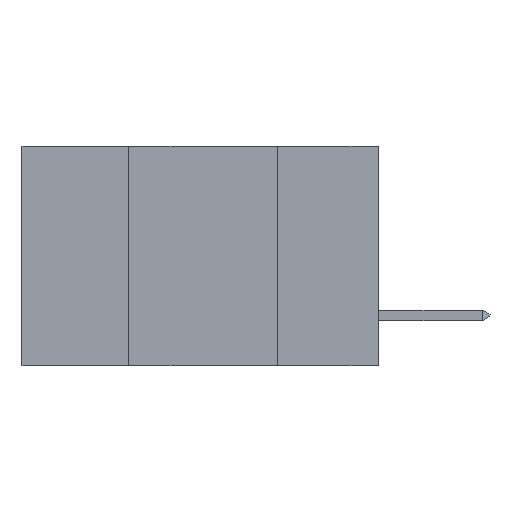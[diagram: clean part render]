
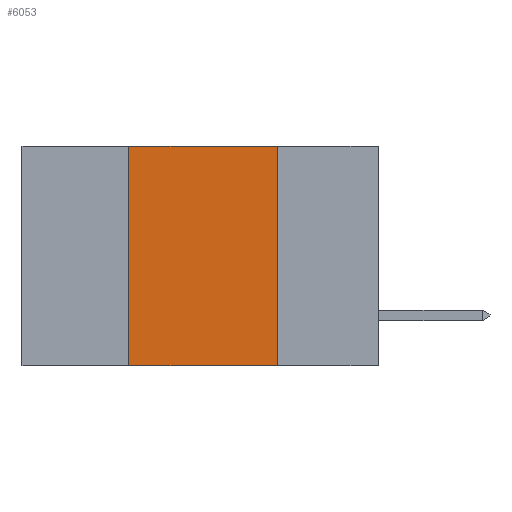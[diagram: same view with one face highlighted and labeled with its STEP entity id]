
A CAD part, left-side view. The second image highlights one B-rep face of the part: STEP entity #6053.
In plain terms, the highlighted planar face has unit normal (-1, 0, 0).
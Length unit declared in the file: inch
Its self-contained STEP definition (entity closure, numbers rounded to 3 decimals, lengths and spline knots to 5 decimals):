
#12 = PLANE ( 'NONE',  #1670 ) ;
#139 = DIRECTION ( 'NONE',  ( 0., 0., -1. ) ) ;
#550 = EDGE_LOOP ( 'NONE', ( #5480, #7150, #6984, #7961 ) ) ;
#715 = FACE_OUTER_BOUND ( 'NONE', #550, .T. ) ;
#751 = LINE ( 'NONE', #3348, #5535 ) ;
#835 = EDGE_CURVE ( 'NONE', #5811, #3957, #4386, .T. ) ;
#1568 = CARTESIAN_POINT ( 'NONE',  ( 0., 0.17, 0. ) ) ;
#1670 = AXIS2_PLACEMENT_3D ( 'NONE', #4110, #5445, #139 ) ;
#2428 = EDGE_CURVE ( 'NONE', #4372, #3389, #8267, .T. ) ;
#3314 = CARTESIAN_POINT ( 'NONE',  ( 0., 0.42, 0. ) ) ;
#3348 = CARTESIAN_POINT ( 'NONE',  ( 0., 0.6, 0. ) ) ;
#3389 = VERTEX_POINT ( 'NONE', #3314 ) ;
#3421 = CARTESIAN_POINT ( 'NONE',  ( 0., 0.6, -0.37 ) ) ;
#3468 = DIRECTION ( 'NONE',  ( 0., -1., 0. ) ) ;
#3649 = DIRECTION ( 'NONE',  ( 0., 0., 1. ) ) ;
#3944 = LINE ( 'NONE', #3421, #8029 ) ;
#3957 = VERTEX_POINT ( 'NONE', #4818 ) ;
#4077 = CARTESIAN_POINT ( 'NONE',  ( 0., 0.42, -0.37 ) ) ;
#4110 = CARTESIAN_POINT ( 'NONE',  ( 0., 0.6, 0. ) ) ;
#4132 = VECTOR ( 'NONE', #3649, 39.37008 ) ;
#4372 = VERTEX_POINT ( 'NONE', #4077 ) ;
#4386 = LINE ( 'NONE', #7805, #6588 ) ;
#4818 = CARTESIAN_POINT ( 'NONE',  ( 0., 0.17, -0.37 ) ) ;
#4830 = EDGE_CURVE ( 'NONE', #4372, #3957, #3944, .T. ) ;
#5445 = DIRECTION ( 'NONE',  ( 1., 0., 0. ) ) ;
#5452 = CARTESIAN_POINT ( 'NONE',  ( 0., 0.42, -0.37 ) ) ;
#5480 = ORIENTED_EDGE ( 'NONE', *, *, #835, .F. ) ;
#5535 = VECTOR ( 'NONE', #7957, 39.37008 ) ;
#5811 = VERTEX_POINT ( 'NONE', #1568 ) ;
#6048 = EDGE_CURVE ( 'NONE', #3389, #5811, #751, .T. ) ;
#6053 = ADVANCED_FACE ( 'NONE', ( #715 ), #12, .F. ) ;
#6588 = VECTOR ( 'NONE', #8452, 39.37008 ) ;
#6984 = ORIENTED_EDGE ( 'NONE', *, *, #2428, .F. ) ;
#7150 = ORIENTED_EDGE ( 'NONE', *, *, #6048, .F. ) ;
#7805 = CARTESIAN_POINT ( 'NONE',  ( 0., 0.17, -0.37 ) ) ;
#7957 = DIRECTION ( 'NONE',  ( 0., -1., 0. ) ) ;
#7961 = ORIENTED_EDGE ( 'NONE', *, *, #4830, .T. ) ;
#8029 = VECTOR ( 'NONE', #3468, 39.37008 ) ;
#8267 = LINE ( 'NONE', #5452, #4132 ) ;
#8452 = DIRECTION ( 'NONE',  ( 0., 0., -1. ) ) ;
